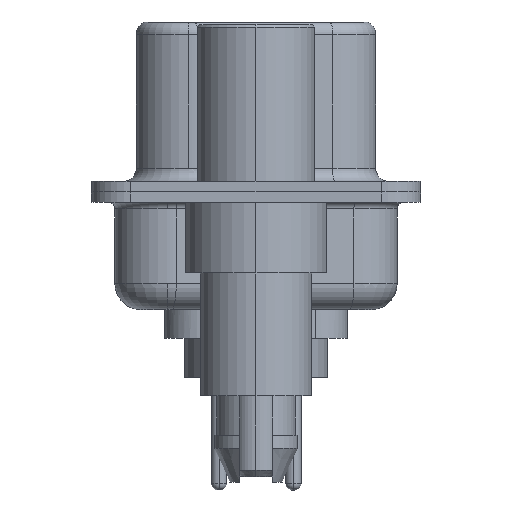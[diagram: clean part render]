
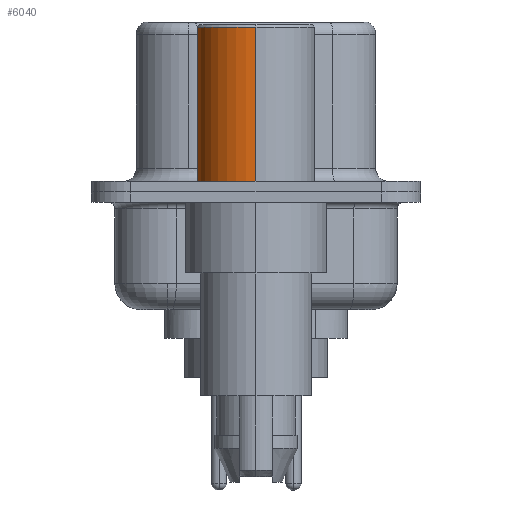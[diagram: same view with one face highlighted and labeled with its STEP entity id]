
A CAD part, left-side view. The second image highlights one B-rep face of the part: STEP entity #6040.
In plain terms, the highlighted cylindrical face has radius 2.25 mm (diameter 4.5 mm), a partial arc.
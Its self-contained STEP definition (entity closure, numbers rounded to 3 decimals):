
#65 = CARTESIAN_POINT ( 'NONE',  ( 0., 0., 0.4 ) ) ;
#380 = LINE ( 'NONE', #12514, #8061 ) ;
#920 = ORIENTED_EDGE ( 'NONE', *, *, #15484, .F. ) ;
#1233 = LINE ( 'NONE', #15592, #7978 ) ;
#1519 = DIRECTION ( 'NONE',  ( 1., 0., 0. ) ) ;
#2163 = EDGE_CURVE ( 'NONE', #4029, #10838, #1233, .T. ) ;
#2293 = CIRCLE ( 'NONE', #15887, 2.25 ) ;
#4029 = VERTEX_POINT ( 'NONE', #9619 ) ;
#4199 = CARTESIAN_POINT ( 'NONE',  ( 0., 0., 6.3 ) ) ;
#4931 = CARTESIAN_POINT ( 'NONE',  ( 2.25, 0., 6.3 ) ) ;
#5633 = DIRECTION ( 'NONE',  ( 1., 0., 0. ) ) ;
#5744 = ORIENTED_EDGE ( 'NONE', *, *, #12685, .F. ) ;
#6040 = ADVANCED_FACE ( 'NONE', ( #16494 ), #16030, .T. ) ;
#6577 = ORIENTED_EDGE ( 'NONE', *, *, #12295, .T. ) ;
#7105 = DIRECTION ( 'NONE',  ( 1., 0., 0. ) ) ;
#7978 = VECTOR ( 'NONE', #8485, 1000. ) ;
#8061 = VECTOR ( 'NONE', #16771, 1000. ) ;
#8485 = DIRECTION ( 'NONE',  ( 0., 0., 1. ) ) ;
#8508 = DIRECTION ( 'NONE',  ( 0., 0., 1. ) ) ;
#9353 = ORIENTED_EDGE ( 'NONE', *, *, #2163, .T. ) ;
#9619 = CARTESIAN_POINT ( 'NONE',  ( -2.25, 0., 0.4 ) ) ;
#9622 = AXIS2_PLACEMENT_3D ( 'NONE', #65, #10145, #1519 ) ;
#10145 = DIRECTION ( 'NONE',  ( 0., 0., 1. ) ) ;
#10838 = VERTEX_POINT ( 'NONE', #15062 ) ;
#11488 = CARTESIAN_POINT ( 'NONE',  ( 0., 0., 0.581 ) ) ;
#11559 = VERTEX_POINT ( 'NONE', #12475 ) ;
#12017 = VERTEX_POINT ( 'NONE', #4931 ) ;
#12295 = EDGE_CURVE ( 'NONE', #11559, #4029, #14408, .T. ) ;
#12475 = CARTESIAN_POINT ( 'NONE',  ( 2.25, 0., 0.4 ) ) ;
#12514 = CARTESIAN_POINT ( 'NONE',  ( 2.25, 0., 0.581 ) ) ;
#12685 = EDGE_CURVE ( 'NONE', #11559, #12017, #380, .T. ) ;
#14300 = DIRECTION ( 'NONE',  ( 0., 0., 1. ) ) ;
#14408 = CIRCLE ( 'NONE', #9622, 2.25 ) ;
#14850 = AXIS2_PLACEMENT_3D ( 'NONE', #11488, #8508, #7105 ) ;
#15062 = CARTESIAN_POINT ( 'NONE',  ( -2.25, 0., 6.3 ) ) ;
#15484 = EDGE_CURVE ( 'NONE', #12017, #10838, #2293, .T. ) ;
#15592 = CARTESIAN_POINT ( 'NONE',  ( -2.25, 0., 0.581 ) ) ;
#15887 = AXIS2_PLACEMENT_3D ( 'NONE', #4199, #14300, #5633 ) ;
#16030 = CYLINDRICAL_SURFACE ( 'NONE', #14850, 2.25 ) ;
#16494 = FACE_OUTER_BOUND ( 'NONE', #17450, .T. ) ;
#16771 = DIRECTION ( 'NONE',  ( 0., 0., 1. ) ) ;
#17450 = EDGE_LOOP ( 'NONE', ( #6577, #9353, #920, #5744 ) ) ;
